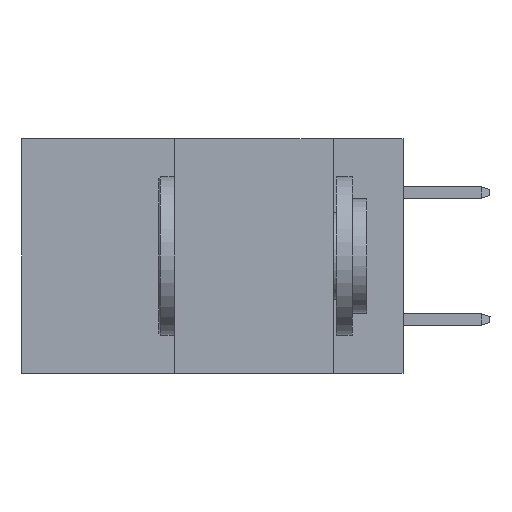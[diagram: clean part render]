
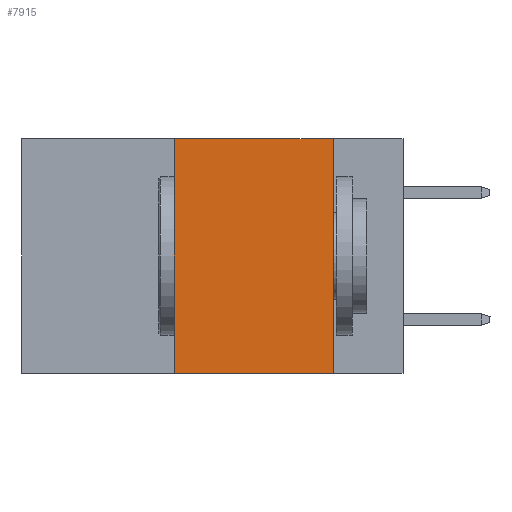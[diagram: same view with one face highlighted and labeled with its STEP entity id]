
A CAD part, left-side view. The second image highlights one B-rep face of the part: STEP entity #7915.
In plain terms, the highlighted planar face has unit normal (-1, 0, 0).
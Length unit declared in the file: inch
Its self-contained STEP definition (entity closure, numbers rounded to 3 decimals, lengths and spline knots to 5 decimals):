
#82 = CARTESIAN_POINT ( 'NONE',  ( 0., 0.11, 0. ) ) ;
#628 = ORIENTED_EDGE ( 'NONE', *, *, #10430, .F. ) ;
#2244 = VERTEX_POINT ( 'NONE', #12814 ) ;
#2285 = VECTOR ( 'NONE', #13988, 39.37008 ) ;
#2364 = VECTOR ( 'NONE', #6602, 39.37008 ) ;
#4044 = CARTESIAN_POINT ( 'NONE',  ( 0., 0.36, 0. ) ) ;
#4102 = ORIENTED_EDGE ( 'NONE', *, *, #14234, .T. ) ;
#4538 = CARTESIAN_POINT ( 'NONE',  ( 0., 0.6, 0. ) ) ;
#4714 = ORIENTED_EDGE ( 'NONE', *, *, #13797, .F. ) ;
#5360 = DIRECTION ( 'NONE',  ( 0., -1., 0. ) ) ;
#5692 = DIRECTION ( 'NONE',  ( 0., 0., -1. ) ) ;
#5781 = VECTOR ( 'NONE', #12539, 39.37008 ) ;
#6058 = CARTESIAN_POINT ( 'NONE',  ( 0., 0.6, 0. ) ) ;
#6365 = CARTESIAN_POINT ( 'NONE',  ( 0., 0.11, 0. ) ) ;
#6602 = DIRECTION ( 'NONE',  ( 0., 0., -1. ) ) ;
#7915 = ADVANCED_FACE ( 'NONE', ( #15513 ), #14416, .F. ) ;
#8293 = VERTEX_POINT ( 'NONE', #10534 ) ;
#9551 = DIRECTION ( 'NONE',  ( 1., 0., 0. ) ) ;
#9720 = EDGE_LOOP ( 'NONE', ( #10073, #4714, #628, #4102 ) ) ;
#9747 = VERTEX_POINT ( 'NONE', #10942 ) ;
#10058 = CARTESIAN_POINT ( 'NONE',  ( 0., 0.6, -0.37 ) ) ;
#10073 = ORIENTED_EDGE ( 'NONE', *, *, #14280, .F. ) ;
#10213 = LINE ( 'NONE', #6365, #2364 ) ;
#10430 = EDGE_CURVE ( 'NONE', #9747, #2244, #12831, .T. ) ;
#10534 = CARTESIAN_POINT ( 'NONE',  ( 0., 0.11, -0.37 ) ) ;
#10942 = CARTESIAN_POINT ( 'NONE',  ( 0., 0.36, -0.37 ) ) ;
#12539 = DIRECTION ( 'NONE',  ( 0., -1., 0. ) ) ;
#12814 = CARTESIAN_POINT ( 'NONE',  ( 0., 0.36, 0. ) ) ;
#12831 = LINE ( 'NONE', #4044, #2285 ) ;
#13485 = VERTEX_POINT ( 'NONE', #82 ) ;
#13797 = EDGE_CURVE ( 'NONE', #2244, #13485, #16273, .T. ) ;
#13988 = DIRECTION ( 'NONE',  ( 0., 0., 1. ) ) ;
#14234 = EDGE_CURVE ( 'NONE', #9747, #8293, #15083, .T. ) ;
#14280 = EDGE_CURVE ( 'NONE', #13485, #8293, #10213, .T. ) ;
#14416 = PLANE ( 'NONE',  #14774 ) ;
#14774 = AXIS2_PLACEMENT_3D ( 'NONE', #4538, #9551, #5692 ) ;
#15083 = LINE ( 'NONE', #10058, #15548 ) ;
#15513 = FACE_OUTER_BOUND ( 'NONE', #9720, .T. ) ;
#15548 = VECTOR ( 'NONE', #5360, 39.37008 ) ;
#16273 = LINE ( 'NONE', #6058, #5781 ) ;
